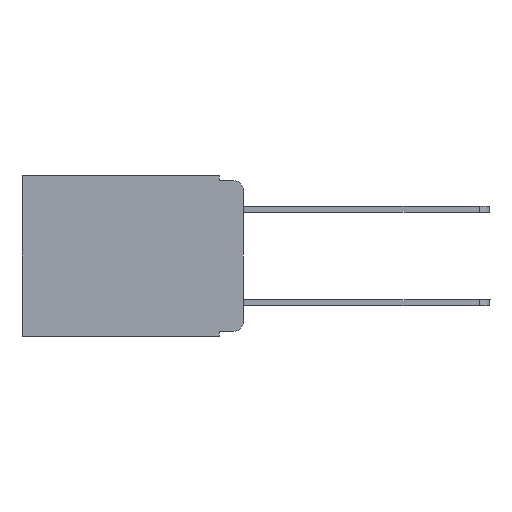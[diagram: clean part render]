
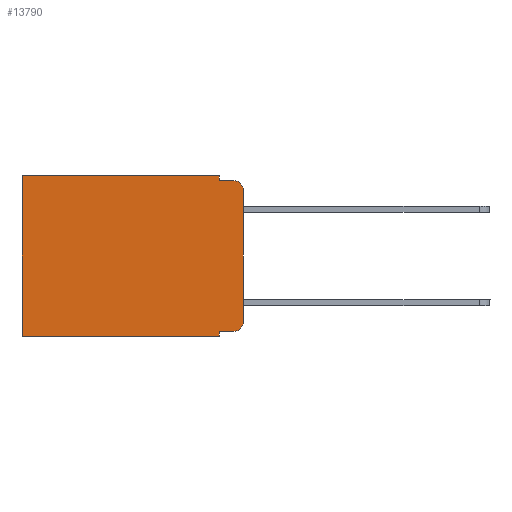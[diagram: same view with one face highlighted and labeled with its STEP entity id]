
A CAD part, left-side view. The second image highlights one B-rep face of the part: STEP entity #13790.
In plain terms, the highlighted planar face has unit normal (-1, 0, 0).
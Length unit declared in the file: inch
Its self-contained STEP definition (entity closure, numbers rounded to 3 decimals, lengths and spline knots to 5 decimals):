
#614 = VECTOR ( 'NONE', #6620, 39.37008 ) ;
#652 = DIRECTION ( 'NONE',  ( 0., -1., 0. ) ) ;
#672 = EDGE_CURVE ( 'NONE', #10710, #10431, #11456, .T. ) ;
#923 = EDGE_CURVE ( 'NONE', #11598, #5654, #1568, .T. ) ;
#1110 = CARTESIAN_POINT ( 'NONE',  ( 0.298, 0.051, -0.01 ) ) ;
#1212 = LINE ( 'NONE', #3012, #10921 ) ;
#1285 = ORIENTED_EDGE ( 'NONE', *, *, #12909, .T. ) ;
#1488 = VERTEX_POINT ( 'NONE', #1698 ) ;
#1568 = LINE ( 'NONE', #9811, #11442 ) ;
#1648 = CARTESIAN_POINT ( 'NONE',  ( 0.298, 0.473, 0. ) ) ;
#1698 = CARTESIAN_POINT ( 'NONE',  ( 0.298, 0.473, -0.343 ) ) ;
#2250 = CARTESIAN_POINT ( 'NONE',  ( 0.298, 0.051, 0. ) ) ;
#2726 = VECTOR ( 'NONE', #12874, 39.37008 ) ;
#3006 = CARTESIAN_POINT ( 'NONE',  ( 0.298, 0., 0. ) ) ;
#3012 = CARTESIAN_POINT ( 'NONE',  ( 0.298, 0.051, -0.01 ) ) ;
#3063 = VERTEX_POINT ( 'NONE', #1648 ) ;
#3287 = CARTESIAN_POINT ( 'NONE',  ( 0.298, 0., -0.03 ) ) ;
#3650 = DIRECTION ( 'NONE',  ( 0., 0., -1. ) ) ;
#3805 = EDGE_CURVE ( 'NONE', #3063, #1488, #4088, .T. ) ;
#4065 = EDGE_CURVE ( 'NONE', #5451, #10431, #4599, .T. ) ;
#4088 = LINE ( 'NONE', #6361, #2726 ) ;
#4334 = DIRECTION ( 'NONE',  ( -1., 0., 0. ) ) ;
#4557 = VERTEX_POINT ( 'NONE', #10454 ) ;
#4568 = VERTEX_POINT ( 'NONE', #6223 ) ;
#4599 = LINE ( 'NONE', #6136, #8044 ) ;
#4810 = PLANE ( 'NONE',  #11811 ) ;
#4815 = CARTESIAN_POINT ( 'NONE',  ( 0.298, 0., 0. ) ) ;
#5443 = EDGE_CURVE ( 'NONE', #5451, #4568, #8348, .T. ) ;
#5451 = VERTEX_POINT ( 'NONE', #3287 ) ;
#5654 = VERTEX_POINT ( 'NONE', #1110 ) ;
#5715 = DIRECTION ( 'NONE',  ( 0., 1., 0. ) ) ;
#5841 = EDGE_CURVE ( 'NONE', #4557, #1488, #7818, .T. ) ;
#5975 = AXIS2_PLACEMENT_3D ( 'NONE', #13736, #6318, #12827 ) ;
#6050 = LINE ( 'NONE', #7964, #10147 ) ;
#6097 = VERTEX_POINT ( 'NONE', #12761 ) ;
#6136 = CARTESIAN_POINT ( 'NONE',  ( 0.298, 0., 0. ) ) ;
#6223 = CARTESIAN_POINT ( 'NONE',  ( 0.298, 0.02, -0.01 ) ) ;
#6318 = DIRECTION ( 'NONE',  ( -1., 0., 0. ) ) ;
#6361 = CARTESIAN_POINT ( 'NONE',  ( 0.298, 0.473, 0. ) ) ;
#6620 = DIRECTION ( 'NONE',  ( 0., 0., -1. ) ) ;
#6711 = CARTESIAN_POINT ( 'NONE',  ( 0.298, 0.051, 0. ) ) ;
#7047 = AXIS2_PLACEMENT_3D ( 'NONE', #11883, #4334, #10763 ) ;
#7155 = DIRECTION ( 'NONE',  ( 0., 0., -1. ) ) ;
#7189 = EDGE_CURVE ( 'NONE', #6097, #10710, #6050, .T. ) ;
#7818 = LINE ( 'NONE', #9083, #11681 ) ;
#7964 = CARTESIAN_POINT ( 'NONE',  ( 0.298, 0.051, -0.333 ) ) ;
#8023 = ORIENTED_EDGE ( 'NONE', *, *, #672, .T. ) ;
#8044 = VECTOR ( 'NONE', #7155, 39.37008 ) ;
#8054 = ORIENTED_EDGE ( 'NONE', *, *, #5443, .T. ) ;
#8168 = ORIENTED_EDGE ( 'NONE', *, *, #4065, .F. ) ;
#8249 = ORIENTED_EDGE ( 'NONE', *, *, #5841, .F. ) ;
#8341 = LINE ( 'NONE', #2250, #614 ) ;
#8348 = CIRCLE ( 'NONE', #7047, 0.02 ) ;
#8520 = DIRECTION ( 'NONE',  ( 0., 0., -1. ) ) ;
#8661 = LINE ( 'NONE', #4815, #9495 ) ;
#9083 = CARTESIAN_POINT ( 'NONE',  ( 0.298, 0., -0.343 ) ) ;
#9311 = DIRECTION ( 'NONE',  ( 1., 0., 0. ) ) ;
#9495 = VECTOR ( 'NONE', #10206, 39.37008 ) ;
#9736 = EDGE_CURVE ( 'NONE', #5654, #4568, #1212, .T. ) ;
#9811 = CARTESIAN_POINT ( 'NONE',  ( 0.298, 0.051, 0. ) ) ;
#10147 = VECTOR ( 'NONE', #652, 39.37008 ) ;
#10206 = DIRECTION ( 'NONE',  ( 0., 1., 0. ) ) ;
#10334 = CARTESIAN_POINT ( 'NONE',  ( 0.298, 0.02, -0.333 ) ) ;
#10376 = CARTESIAN_POINT ( 'NONE',  ( 0.298, 0., -0.313 ) ) ;
#10431 = VERTEX_POINT ( 'NONE', #10376 ) ;
#10454 = CARTESIAN_POINT ( 'NONE',  ( 0.298, 0.051, -0.343 ) ) ;
#10469 = ORIENTED_EDGE ( 'NONE', *, *, #7189, .T. ) ;
#10622 = DIRECTION ( 'NONE',  ( 0., -1., 0. ) ) ;
#10710 = VERTEX_POINT ( 'NONE', #10334 ) ;
#10763 = DIRECTION ( 'NONE',  ( 0., 0., -1. ) ) ;
#10921 = VECTOR ( 'NONE', #10622, 39.37008 ) ;
#10988 = ORIENTED_EDGE ( 'NONE', *, *, #9736, .F. ) ;
#11442 = VECTOR ( 'NONE', #3650, 39.37008 ) ;
#11456 = CIRCLE ( 'NONE', #5975, 0.02 ) ;
#11598 = VERTEX_POINT ( 'NONE', #6711 ) ;
#11680 = ORIENTED_EDGE ( 'NONE', *, *, #3805, .T. ) ;
#11681 = VECTOR ( 'NONE', #5715, 39.37008 ) ;
#11750 = EDGE_LOOP ( 'NONE', ( #8168, #8054, #10988, #12539, #1285, #11680, #8249, #12851, #10469, #8023 ) ) ;
#11811 = AXIS2_PLACEMENT_3D ( 'NONE', #3006, #9311, #8520 ) ;
#11883 = CARTESIAN_POINT ( 'NONE',  ( 0.298, 0.02, -0.03 ) ) ;
#12324 = FACE_OUTER_BOUND ( 'NONE', #11750, .T. ) ;
#12539 = ORIENTED_EDGE ( 'NONE', *, *, #923, .F. ) ;
#12726 = EDGE_CURVE ( 'NONE', #6097, #4557, #8341, .T. ) ;
#12761 = CARTESIAN_POINT ( 'NONE',  ( 0.298, 0.051, -0.333 ) ) ;
#12827 = DIRECTION ( 'NONE',  ( 0., 0., -1. ) ) ;
#12851 = ORIENTED_EDGE ( 'NONE', *, *, #12726, .F. ) ;
#12874 = DIRECTION ( 'NONE',  ( 0., 0., -1. ) ) ;
#12909 = EDGE_CURVE ( 'NONE', #11598, #3063, #8661, .T. ) ;
#13736 = CARTESIAN_POINT ( 'NONE',  ( 0.298, 0.02, -0.313 ) ) ;
#13790 = ADVANCED_FACE ( 'NONE', ( #12324 ), #4810, .F. ) ;
